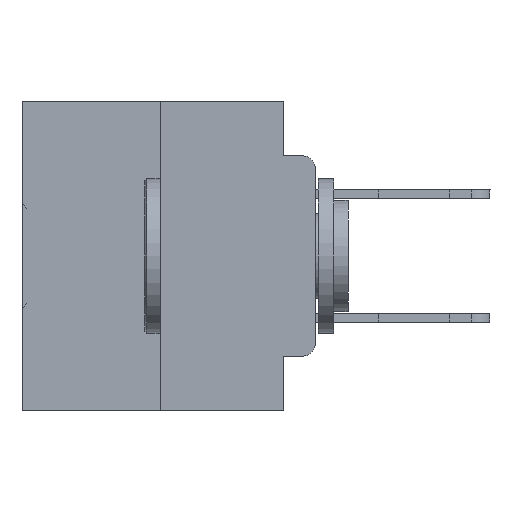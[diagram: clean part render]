
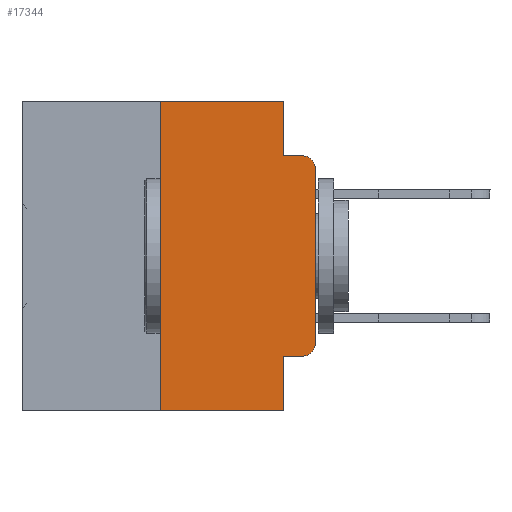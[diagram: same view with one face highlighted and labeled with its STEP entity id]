
A CAD part, left-side view. The second image highlights one B-rep face of the part: STEP entity #17344.
In plain terms, the highlighted planar face has unit normal (-1, 0, 0).
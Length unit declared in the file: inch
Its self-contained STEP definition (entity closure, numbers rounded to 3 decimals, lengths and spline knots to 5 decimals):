
#294 = EDGE_LOOP ( 'NONE', ( #24878, #4116, #11593, #5682, #30591, #28746, #31808, #14406, #8181, #28117 ) ) ;
#313 = LINE ( 'NONE', #32516, #5891 ) ;
#470 = CARTESIAN_POINT ( 'NONE',  ( 0., 0., -0.3915 ) ) ;
#703 = CARTESIAN_POINT ( 'NONE',  ( 0., 0.051, 0. ) ) ;
#1648 = DIRECTION ( 'NONE',  ( 0., 0., -1. ) ) ;
#1677 = VERTEX_POINT ( 'NONE', #31619 ) ;
#2219 = CARTESIAN_POINT ( 'NONE',  ( 0., 0.051, -0.0885 ) ) ;
#2958 = DIRECTION ( 'NONE',  ( 0., -1., 0. ) ) ;
#3270 = VERTEX_POINT ( 'NONE', #12063 ) ;
#3565 = VECTOR ( 'NONE', #2958, 39.37008 ) ;
#3740 = PLANE ( 'NONE',  #26997 ) ;
#3763 = EDGE_CURVE ( 'NONE', #3270, #7618, #26152, .T. ) ;
#4116 = ORIENTED_EDGE ( 'NONE', *, *, #29760, .T. ) ;
#4288 = CARTESIAN_POINT ( 'NONE',  ( 0., 0.25, 0. ) ) ;
#4486 = VERTEX_POINT ( 'NONE', #10695 ) ;
#4617 = EDGE_CURVE ( 'NONE', #7618, #15306, #26609, .T. ) ;
#5682 = ORIENTED_EDGE ( 'NONE', *, *, #15577, .F. ) ;
#5891 = VECTOR ( 'NONE', #7825, 39.37008 ) ;
#5929 = VERTEX_POINT ( 'NONE', #470 ) ;
#6481 = DIRECTION ( 'NONE',  ( 1., 0., 0. ) ) ;
#7599 = VECTOR ( 'NONE', #34778, 39.37008 ) ;
#7618 = VERTEX_POINT ( 'NONE', #27646 ) ;
#7825 = DIRECTION ( 'NONE',  ( 0., -1., 0. ) ) ;
#8181 = ORIENTED_EDGE ( 'NONE', *, *, #21212, .T. ) ;
#8852 = DIRECTION ( 'NONE',  ( 0., 0., -1. ) ) ;
#9650 = CARTESIAN_POINT ( 'NONE',  ( 0., 0., 0. ) ) ;
#9745 = VECTOR ( 'NONE', #26229, 39.37008 ) ;
#10190 = CARTESIAN_POINT ( 'NONE',  ( 0., 0.051, -0.0885 ) ) ;
#10226 = AXIS2_PLACEMENT_3D ( 'NONE', #29919, #19389, #18516 ) ;
#10390 = VECTOR ( 'NONE', #12595, 39.37008 ) ;
#10695 = CARTESIAN_POINT ( 'NONE',  ( 0., 0.051, -0.5 ) ) ;
#10826 = CARTESIAN_POINT ( 'NONE',  ( 0., 0.473, 0. ) ) ;
#10977 = EDGE_CURVE ( 'NONE', #3270, #4486, #28109, .T. ) ;
#11593 = ORIENTED_EDGE ( 'NONE', *, *, #27295, .F. ) ;
#12063 = CARTESIAN_POINT ( 'NONE',  ( 0., 0.25, -0.5 ) ) ;
#12142 = DIRECTION ( 'NONE',  ( 0., 0., 1. ) ) ;
#12322 = LINE ( 'NONE', #9650, #9745 ) ;
#12595 = DIRECTION ( 'NONE',  ( 0., 0., -1. ) ) ;
#13979 = DIRECTION ( 'NONE',  ( 0., 0., -1. ) ) ;
#14302 = VECTOR ( 'NONE', #1648, 39.37008 ) ;
#14406 = ORIENTED_EDGE ( 'NONE', *, *, #16903, .F. ) ;
#14744 = VERTEX_POINT ( 'NONE', #22439 ) ;
#14972 = CARTESIAN_POINT ( 'NONE',  ( 0., 0.051, 0. ) ) ;
#15251 = CIRCLE ( 'NONE', #34150, 0.02 ) ;
#15306 = VERTEX_POINT ( 'NONE', #703 ) ;
#15577 = EDGE_CURVE ( 'NONE', #15306, #32361, #25017, .T. ) ;
#16766 = LINE ( 'NONE', #23801, #10390 ) ;
#16903 = EDGE_CURVE ( 'NONE', #34000, #4486, #16766, .T. ) ;
#17344 = ADVANCED_FACE ( 'NONE', ( #27452 ), #3740, .F. ) ;
#18479 = CARTESIAN_POINT ( 'NONE',  ( 0., 0.051, -0.4115 ) ) ;
#18516 = DIRECTION ( 'NONE',  ( 0., 0., -1. ) ) ;
#19389 = DIRECTION ( 'NONE',  ( -1., 0., 0. ) ) ;
#19480 = DIRECTION ( 'NONE',  ( -1., 0., 0. ) ) ;
#19999 = VECTOR ( 'NONE', #29099, 39.37008 ) ;
#20318 = CARTESIAN_POINT ( 'NONE',  ( 0., 0., -0.1085 ) ) ;
#20605 = VECTOR ( 'NONE', #12142, 39.37008 ) ;
#20656 = CARTESIAN_POINT ( 'NONE',  ( 0., 0.473, -0.5 ) ) ;
#21212 = EDGE_CURVE ( 'NONE', #34000, #1677, #313, .T. ) ;
#22439 = CARTESIAN_POINT ( 'NONE',  ( 0., 0.02, -0.0885 ) ) ;
#22769 = CARTESIAN_POINT ( 'NONE',  ( 0., 0.473, 0. ) ) ;
#23801 = CARTESIAN_POINT ( 'NONE',  ( 0., 0.051, 0. ) ) ;
#23915 = CIRCLE ( 'NONE', #10226, 0.02 ) ;
#24878 = ORIENTED_EDGE ( 'NONE', *, *, #33803, .T. ) ;
#25017 = LINE ( 'NONE', #14972, #14302 ) ;
#26152 = LINE ( 'NONE', #4288, #20605 ) ;
#26229 = DIRECTION ( 'NONE',  ( 0., 0., 1. ) ) ;
#26609 = LINE ( 'NONE', #10826, #3565 ) ;
#26997 = AXIS2_PLACEMENT_3D ( 'NONE', #22769, #6481, #8852 ) ;
#27295 = EDGE_CURVE ( 'NONE', #32361, #14744, #34032, .T. ) ;
#27452 = FACE_OUTER_BOUND ( 'NONE', #294, .T. ) ;
#27646 = CARTESIAN_POINT ( 'NONE',  ( 0., 0.25, 0. ) ) ;
#28109 = LINE ( 'NONE', #20656, #19999 ) ;
#28117 = ORIENTED_EDGE ( 'NONE', *, *, #31254, .T. ) ;
#28746 = ORIENTED_EDGE ( 'NONE', *, *, #3763, .F. ) ;
#29099 = DIRECTION ( 'NONE',  ( 0., -1., 0. ) ) ;
#29760 = EDGE_CURVE ( 'NONE', #30792, #14744, #23915, .T. ) ;
#29919 = CARTESIAN_POINT ( 'NONE',  ( 0., 0.02, -0.1085 ) ) ;
#30591 = ORIENTED_EDGE ( 'NONE', *, *, #4617, .F. ) ;
#30792 = VERTEX_POINT ( 'NONE', #20318 ) ;
#31254 = EDGE_CURVE ( 'NONE', #1677, #5929, #15251, .T. ) ;
#31619 = CARTESIAN_POINT ( 'NONE',  ( 0., 0.02, -0.4115 ) ) ;
#31808 = ORIENTED_EDGE ( 'NONE', *, *, #10977, .T. ) ;
#32361 = VERTEX_POINT ( 'NONE', #10190 ) ;
#32516 = CARTESIAN_POINT ( 'NONE',  ( 0., 0.051, -0.4115 ) ) ;
#33074 = CARTESIAN_POINT ( 'NONE',  ( 0., 0.02, -0.3915 ) ) ;
#33803 = EDGE_CURVE ( 'NONE', #5929, #30792, #12322, .T. ) ;
#34000 = VERTEX_POINT ( 'NONE', #18479 ) ;
#34032 = LINE ( 'NONE', #2219, #7599 ) ;
#34150 = AXIS2_PLACEMENT_3D ( 'NONE', #33074, #19480, #13979 ) ;
#34778 = DIRECTION ( 'NONE',  ( 0., -1., 0. ) ) ;
